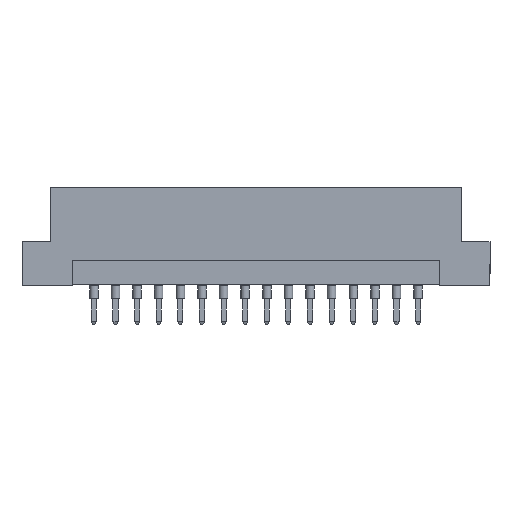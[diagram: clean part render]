
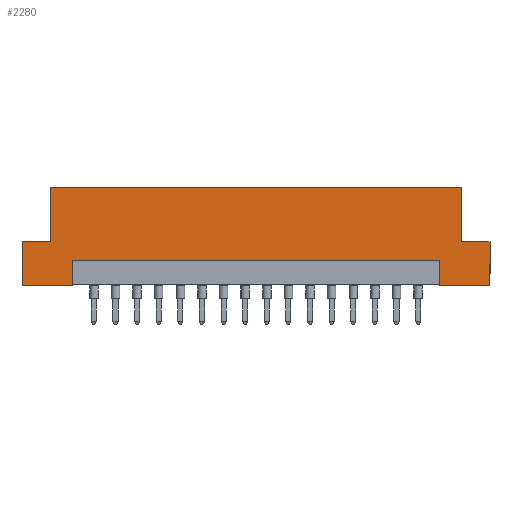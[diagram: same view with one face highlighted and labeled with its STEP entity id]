
A CAD part, front view. The second image highlights one B-rep face of the part: STEP entity #2280.
In plain terms, the highlighted planar face has unit normal (0, -1, 0).
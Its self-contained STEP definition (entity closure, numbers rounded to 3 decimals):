
#137 = EDGE_CURVE ( 'NONE', #5481, #1392, #2576, .T. ) ;
#241 = ORIENTED_EDGE ( 'NONE', *, *, #3225, .F. ) ;
#272 = VECTOR ( 'NONE', #2959, 1000. ) ;
#367 = CARTESIAN_POINT ( 'NONE',  ( 27.5, -4.3, 11.6 ) ) ;
#389 = CARTESIAN_POINT ( 'NONE',  ( -21.6, -4.3, 0.2 ) ) ;
#403 = CARTESIAN_POINT ( 'NONE',  ( -27.5, -4.3, 0. ) ) ;
#462 = LINE ( 'NONE', #7012, #5468 ) ;
#464 = LINE ( 'NONE', #389, #3241 ) ;
#478 = ORIENTED_EDGE ( 'NONE', *, *, #5410, .F. ) ;
#520 = VECTOR ( 'NONE', #5434, 1000. ) ;
#531 = VERTEX_POINT ( 'NONE', #6443 ) ;
#625 = VERTEX_POINT ( 'NONE', #3081 ) ;
#763 = LINE ( 'NONE', #2408, #520 ) ;
#803 = EDGE_CURVE ( 'NONE', #625, #3608, #4482, .T. ) ;
#878 = VECTOR ( 'NONE', #3550, 1000. ) ;
#1023 = VECTOR ( 'NONE', #2091, 1000. ) ;
#1026 = CARTESIAN_POINT ( 'NONE',  ( -27.5, -4.3, 5.2 ) ) ;
#1201 = VERTEX_POINT ( 'NONE', #2481 ) ;
#1270 = CARTESIAN_POINT ( 'NONE',  ( -27.5, -4.3, 5.2 ) ) ;
#1392 = VERTEX_POINT ( 'NONE', #403 ) ;
#1554 = DIRECTION ( 'NONE',  ( 1., 0., 0. ) ) ;
#1619 = ORIENTED_EDGE ( 'NONE', *, *, #2315, .F. ) ;
#1634 = VERTEX_POINT ( 'NONE', #5567 ) ;
#1741 = CARTESIAN_POINT ( 'NONE',  ( -21.6, -4.3, 0. ) ) ;
#1954 = DIRECTION ( 'NONE',  ( 1., 0., 0. ) ) ;
#2091 = DIRECTION ( 'NONE',  ( 0., 0., -1. ) ) ;
#2171 = LINE ( 'NONE', #367, #1023 ) ;
#2280 = ADVANCED_FACE ( 'NONE', ( #5773 ), #2686, .F. ) ;
#2315 = EDGE_CURVE ( 'NONE', #5481, #7059, #5045, .T. ) ;
#2322 = LINE ( 'NONE', #4724, #878 ) ;
#2356 = ORIENTED_EDGE ( 'NONE', *, *, #4629, .T. ) ;
#2408 = CARTESIAN_POINT ( 'NONE',  ( 21.6, -4.3, 0.2 ) ) ;
#2465 = VERTEX_POINT ( 'NONE', #4599 ) ;
#2470 = EDGE_CURVE ( 'NONE', #2465, #3058, #2322, .T. ) ;
#2481 = CARTESIAN_POINT ( 'NONE',  ( 21.6, -4.3, 3. ) ) ;
#2576 = LINE ( 'NONE', #6182, #6657 ) ;
#2630 = VERTEX_POINT ( 'NONE', #3748 ) ;
#2662 = EDGE_CURVE ( 'NONE', #531, #3058, #462, .T. ) ;
#2686 = PLANE ( 'NONE',  #3726 ) ;
#2903 = ORIENTED_EDGE ( 'NONE', *, *, #4323, .F. ) ;
#2959 = DIRECTION ( 'NONE',  ( 1., 0., 0. ) ) ;
#3032 = CARTESIAN_POINT ( 'NONE',  ( -24.2, -4.3, 5.2 ) ) ;
#3058 = VERTEX_POINT ( 'NONE', #3351 ) ;
#3081 = CARTESIAN_POINT ( 'NONE',  ( 21.6, -4.3, 0. ) ) ;
#3218 = DIRECTION ( 'NONE',  ( 1., 0., 0. ) ) ;
#3225 = EDGE_CURVE ( 'NONE', #7059, #531, #6007, .T. ) ;
#3241 = VECTOR ( 'NONE', #5177, 1000. ) ;
#3305 = ORIENTED_EDGE ( 'NONE', *, *, #2470, .T. ) ;
#3336 = ORIENTED_EDGE ( 'NONE', *, *, #3346, .T. ) ;
#3346 = EDGE_CURVE ( 'NONE', #1392, #6539, #7377, .T. ) ;
#3351 = CARTESIAN_POINT ( 'NONE',  ( 24.2, -4.3, 11.6 ) ) ;
#3492 = CARTESIAN_POINT ( 'NONE',  ( 27.5, -4.3, 0. ) ) ;
#3550 = DIRECTION ( 'NONE',  ( 0., 0., 1. ) ) ;
#3608 = VERTEX_POINT ( 'NONE', #3492 ) ;
#3691 = DIRECTION ( 'NONE',  ( 0., 0., -1. ) ) ;
#3726 = AXIS2_PLACEMENT_3D ( 'NONE', #6360, #5694, #5124 ) ;
#3748 = CARTESIAN_POINT ( 'NONE',  ( 27.5, -4.3, 5.2 ) ) ;
#3799 = CARTESIAN_POINT ( 'NONE',  ( 27.5, -4.3, 5.2 ) ) ;
#3865 = DIRECTION ( 'NONE',  ( 1., 0., 0. ) ) ;
#4171 = LINE ( 'NONE', #5903, #272 ) ;
#4323 = EDGE_CURVE ( 'NONE', #2465, #2630, #5444, .T. ) ;
#4356 = VECTOR ( 'NONE', #1954, 1000. ) ;
#4430 = VECTOR ( 'NONE', #6405, 1000. ) ;
#4482 = LINE ( 'NONE', #7388, #6905 ) ;
#4560 = ORIENTED_EDGE ( 'NONE', *, *, #2662, .F. ) ;
#4599 = CARTESIAN_POINT ( 'NONE',  ( 24.2, -4.3, 5.2 ) ) ;
#4629 = EDGE_CURVE ( 'NONE', #1634, #1201, #4171, .T. ) ;
#4633 = CARTESIAN_POINT ( 'NONE',  ( -24.2, -4.3, 5.2 ) ) ;
#4668 = ORIENTED_EDGE ( 'NONE', *, *, #6266, .F. ) ;
#4724 = CARTESIAN_POINT ( 'NONE',  ( 24.2, -4.3, 5.2 ) ) ;
#4735 = EDGE_CURVE ( 'NONE', #625, #1201, #763, .T. ) ;
#4775 = ORIENTED_EDGE ( 'NONE', *, *, #4735, .F. ) ;
#4973 = VECTOR ( 'NONE', #3865, 1000. ) ;
#5045 = LINE ( 'NONE', #1026, #4973 ) ;
#5124 = DIRECTION ( 'NONE',  ( -1., 0., 0. ) ) ;
#5177 = DIRECTION ( 'NONE',  ( 0., 0., -1. ) ) ;
#5410 = EDGE_CURVE ( 'NONE', #1634, #6539, #464, .T. ) ;
#5434 = DIRECTION ( 'NONE',  ( 0., 0., 1. ) ) ;
#5444 = LINE ( 'NONE', #3799, #4356 ) ;
#5468 = VECTOR ( 'NONE', #7165, 1000. ) ;
#5481 = VERTEX_POINT ( 'NONE', #1270 ) ;
#5500 = ORIENTED_EDGE ( 'NONE', *, *, #137, .T. ) ;
#5567 = CARTESIAN_POINT ( 'NONE',  ( -21.6, -4.3, 3. ) ) ;
#5694 = DIRECTION ( 'NONE',  ( 0., 1., 0. ) ) ;
#5720 = VECTOR ( 'NONE', #3218, 1000. ) ;
#5773 = FACE_OUTER_BOUND ( 'NONE', #7300, .T. ) ;
#5903 = CARTESIAN_POINT ( 'NONE',  ( -21.6, -4.3, 3. ) ) ;
#6007 = LINE ( 'NONE', #3032, #4430 ) ;
#6160 = CARTESIAN_POINT ( 'NONE',  ( 27.5, -4.3, 0. ) ) ;
#6182 = CARTESIAN_POINT ( 'NONE',  ( -27.5, -4.3, 11.6 ) ) ;
#6266 = EDGE_CURVE ( 'NONE', #2630, #3608, #2171, .T. ) ;
#6360 = CARTESIAN_POINT ( 'NONE',  ( 27.5, -4.3, 11.6 ) ) ;
#6405 = DIRECTION ( 'NONE',  ( 0., 0., 1. ) ) ;
#6443 = CARTESIAN_POINT ( 'NONE',  ( -24.2, -4.3, 11.6 ) ) ;
#6539 = VERTEX_POINT ( 'NONE', #1741 ) ;
#6657 = VECTOR ( 'NONE', #3691, 1000. ) ;
#6905 = VECTOR ( 'NONE', #1554, 1000. ) ;
#7012 = CARTESIAN_POINT ( 'NONE',  ( 27.5, -4.3, 11.6 ) ) ;
#7059 = VERTEX_POINT ( 'NONE', #4633 ) ;
#7165 = DIRECTION ( 'NONE',  ( 1., 0., 0. ) ) ;
#7300 = EDGE_LOOP ( 'NONE', ( #2356, #4775, #7332, #4668, #2903, #3305, #4560, #241, #1619, #5500, #3336, #478 ) ) ;
#7332 = ORIENTED_EDGE ( 'NONE', *, *, #803, .T. ) ;
#7377 = LINE ( 'NONE', #6160, #5720 ) ;
#7388 = CARTESIAN_POINT ( 'NONE',  ( 27.5, -4.3, 0. ) ) ;
